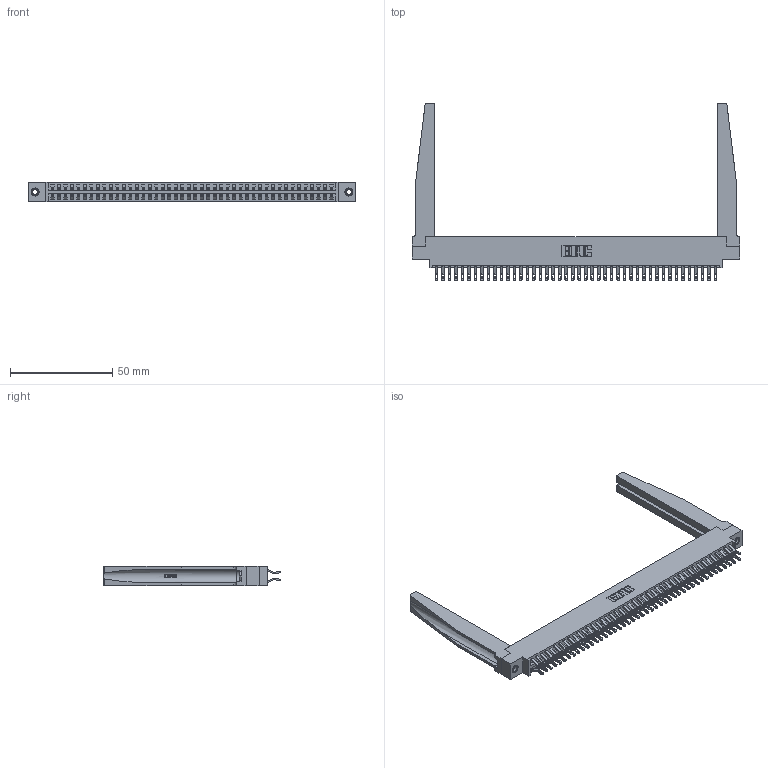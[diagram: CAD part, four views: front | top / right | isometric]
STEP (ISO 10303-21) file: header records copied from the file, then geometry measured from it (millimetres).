
FILE_DESCRIPTION (( 'STEP AP203' ), '1' );
FILE_NAME ('396-088-555-878.STEP', '2019-11-02T15:15:51', ( '' ), ( '' ), 'SwSTEP 2.0', 'SolidWorks 2016', '' );
FILE_SCHEMA (( 'CONFIG_CONTROL_DESIGN' ));
Length unit declared in the file: inch
Products named in the file (5): 346 Part_0.170 Offset - 0.156 Dia-TH; 345-292-001_555 Tail; 346-220-078_345-220-078; 345-250-001_345-250-001-102; 396-088-555-878
Assembly tree (93 placements, depth 2):
  396-088-555-878
    346 Part_0.170 Offset - 0.156 Dia-TH
    345-292-001_555 Tail  x88
    346-220-078_345-220-078  x2
    345-250-001_345-250-001-102  x2
Bounding box: 160.27 x 86.74 x 9.4 mm (x, y, z)
Volume: 22653.7 mm3; surface area: 29300.8 mm2
Topology: 93 solids, 93 shells, 5464 faces, 17053 edges, 11358 vertices
Faces by surface type: plane 3126, cylinder 2286, bspline 36, cone 12, torus 4
Entity records: 33652 total; most frequent: CARTESIAN_POINT 6517, ORIENTED_EDGE 5310, DIRECTION 4749, EDGE_CURVE 2655, VECTOR 2233, LINE 2233, VERTEX_POINT 1764, AXIS2_PLACEMENT_3D 1258
